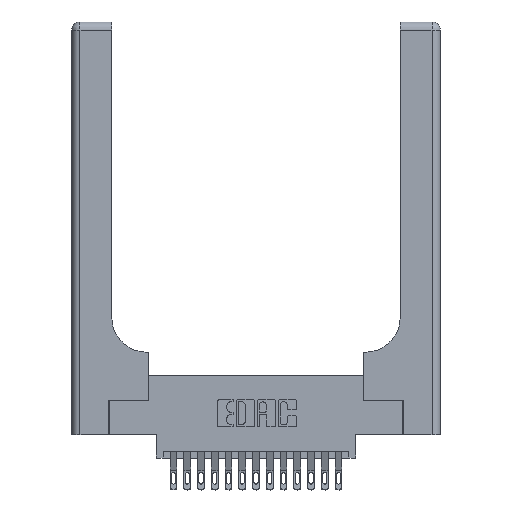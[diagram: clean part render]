
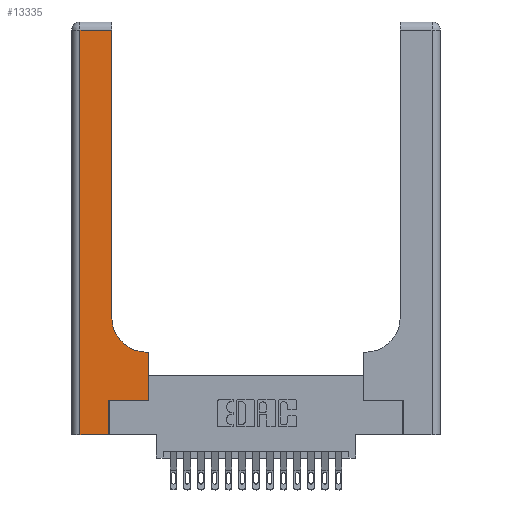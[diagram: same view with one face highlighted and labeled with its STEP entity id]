
A CAD part, top view. The second image highlights one B-rep face of the part: STEP entity #13335.
In plain terms, the highlighted planar face has unit normal (0, 0, 1).
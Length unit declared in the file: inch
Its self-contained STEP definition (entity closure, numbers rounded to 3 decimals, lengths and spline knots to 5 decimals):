
#1 = VECTOR ( 'NONE', #3324, 39.37008 ) ;
#197 = LINE ( 'NONE', #3834, #3309 ) ;
#246 = ORIENTED_EDGE ( 'NONE', *, *, #11885, .T. ) ;
#361 = DIRECTION ( 'NONE',  ( 1., 0., 0. ) ) ;
#392 = DIRECTION ( 'NONE',  ( 0., 1., 0. ) ) ;
#1125 = CARTESIAN_POINT ( 'NONE',  ( 0.5415, 0.6, 0.37 ) ) ;
#1129 = PLANE ( 'NONE',  #8387 ) ;
#1445 = CARTESIAN_POINT ( 'NONE',  ( 0.269, 0.25, 0.37 ) ) ;
#2044 = CARTESIAN_POINT ( 'NONE',  ( 0.5415, 0.85, 0.37 ) ) ;
#2123 = EDGE_CURVE ( 'NONE', #8630, #7071, #16286, .T. ) ;
#2138 = CARTESIAN_POINT ( 'NONE',  ( 0.269, 0., 0.37 ) ) ;
#2333 = CARTESIAN_POINT ( 'NONE',  ( 0.2915, 0.85, 0.37 ) ) ;
#2960 = DIRECTION ( 'NONE',  ( 1., 0., 0. ) ) ;
#3099 = EDGE_CURVE ( 'NONE', #7071, #17061, #6461, .T. ) ;
#3209 = CARTESIAN_POINT ( 'NONE',  ( 0.5585, 0.6, 0.37 ) ) ;
#3309 = VECTOR ( 'NONE', #14486, 39.37008 ) ;
#3324 = DIRECTION ( 'NONE',  ( 0., -1., 0. ) ) ;
#3732 = DIRECTION ( 'NONE',  ( -1., 0., 0. ) ) ;
#3834 = CARTESIAN_POINT ( 'NONE',  ( 0.2915, 0.6, 0.37 ) ) ;
#4748 = CARTESIAN_POINT ( 'NONE',  ( 0.269, 0.25, 0.37 ) ) ;
#4869 = CARTESIAN_POINT ( 'NONE',  ( 0.5585, 0.25, 0.37 ) ) ;
#5090 = CARTESIAN_POINT ( 'NONE',  ( 0.5585, 0.25, 0.37 ) ) ;
#5137 = CARTESIAN_POINT ( 'NONE',  ( 0., 2.94, 0.37 ) ) ;
#5686 = CARTESIAN_POINT ( 'NONE',  ( 0.06, 2.94, 0.37 ) ) ;
#5844 = LINE ( 'NONE', #4748, #17317 ) ;
#6461 = LINE ( 'NONE', #15744, #18871 ) ;
#6571 = EDGE_CURVE ( 'NONE', #16736, #7818, #13984, .T. ) ;
#7071 = VERTEX_POINT ( 'NONE', #2138 ) ;
#7245 = DIRECTION ( 'NONE',  ( 0., 0., -1. ) ) ;
#7269 = VERTEX_POINT ( 'NONE', #5686 ) ;
#7566 = ORIENTED_EDGE ( 'NONE', *, *, #13179, .T. ) ;
#7678 = ORIENTED_EDGE ( 'NONE', *, *, #15500, .T. ) ;
#7818 = VERTEX_POINT ( 'NONE', #7953 ) ;
#7860 = EDGE_LOOP ( 'NONE', ( #19575, #9196, #7566, #16775, #11547, #7678, #11458, #246, #11186 ) ) ;
#7953 = CARTESIAN_POINT ( 'NONE',  ( 0.2915, 2.94, 0.37 ) ) ;
#8075 = DIRECTION ( 'NONE',  ( 0., 1., 0. ) ) ;
#8101 = LINE ( 'NONE', #12263, #1 ) ;
#8387 = AXIS2_PLACEMENT_3D ( 'NONE', #15844, #7245, #3732 ) ;
#8417 = EDGE_CURVE ( 'NONE', #9008, #19215, #10811, .T. ) ;
#8630 = VERTEX_POINT ( 'NONE', #15170 ) ;
#9008 = VERTEX_POINT ( 'NONE', #4869 ) ;
#9196 = ORIENTED_EDGE ( 'NONE', *, *, #9766, .T. ) ;
#9766 = EDGE_CURVE ( 'NONE', #7818, #7269, #16945, .T. ) ;
#10811 = LINE ( 'NONE', #5090, #13913 ) ;
#11080 = DIRECTION ( 'NONE',  ( -1., 0., 0. ) ) ;
#11186 = ORIENTED_EDGE ( 'NONE', *, *, #15613, .T. ) ;
#11349 = DIRECTION ( 'NONE',  ( 0., 0., -1. ) ) ;
#11458 = ORIENTED_EDGE ( 'NONE', *, *, #8417, .T. ) ;
#11547 = ORIENTED_EDGE ( 'NONE', *, *, #3099, .T. ) ;
#11885 = EDGE_CURVE ( 'NONE', #19215, #16889, #197, .T. ) ;
#12263 = CARTESIAN_POINT ( 'NONE',  ( 0.06, 3., 0.37 ) ) ;
#12553 = VECTOR ( 'NONE', #392, 39.37008 ) ;
#12892 = DIRECTION ( 'NONE',  ( 1., 0., 0. ) ) ;
#13179 = EDGE_CURVE ( 'NONE', #7269, #8630, #8101, .T. ) ;
#13335 = ADVANCED_FACE ( 'NONE', ( #17405 ), #1129, .F. ) ;
#13508 = CIRCLE ( 'NONE', #18133, 0.25 ) ;
#13913 = VECTOR ( 'NONE', #18911, 39.37008 ) ;
#13984 = LINE ( 'NONE', #15155, #12553 ) ;
#14486 = DIRECTION ( 'NONE',  ( -1., 0., 0. ) ) ;
#15155 = CARTESIAN_POINT ( 'NONE',  ( 0.2915, 3., 0.37 ) ) ;
#15170 = CARTESIAN_POINT ( 'NONE',  ( 0.06, 0., 0.37 ) ) ;
#15500 = EDGE_CURVE ( 'NONE', #17061, #9008, #5844, .T. ) ;
#15613 = EDGE_CURVE ( 'NONE', #16889, #16736, #13508, .T. ) ;
#15744 = CARTESIAN_POINT ( 'NONE',  ( 0.269, 0., 0.37 ) ) ;
#15844 = CARTESIAN_POINT ( 'NONE',  ( 0., 3., 0.37 ) ) ;
#16286 = LINE ( 'NONE', #16605, #18680 ) ;
#16605 = CARTESIAN_POINT ( 'NONE',  ( 0., 0., 0.37 ) ) ;
#16736 = VERTEX_POINT ( 'NONE', #2333 ) ;
#16775 = ORIENTED_EDGE ( 'NONE', *, *, #2123, .T. ) ;
#16889 = VERTEX_POINT ( 'NONE', #1125 ) ;
#16945 = LINE ( 'NONE', #5137, #17896 ) ;
#17061 = VERTEX_POINT ( 'NONE', #1445 ) ;
#17317 = VECTOR ( 'NONE', #361, 39.37008 ) ;
#17405 = FACE_OUTER_BOUND ( 'NONE', #7860, .T. ) ;
#17896 = VECTOR ( 'NONE', #11080, 39.37008 ) ;
#18133 = AXIS2_PLACEMENT_3D ( 'NONE', #2044, #11349, #12892 ) ;
#18680 = VECTOR ( 'NONE', #2960, 39.37008 ) ;
#18871 = VECTOR ( 'NONE', #8075, 39.37008 ) ;
#18911 = DIRECTION ( 'NONE',  ( 0., 1., 0. ) ) ;
#19215 = VERTEX_POINT ( 'NONE', #3209 ) ;
#19575 = ORIENTED_EDGE ( 'NONE', *, *, #6571, .T. ) ;
